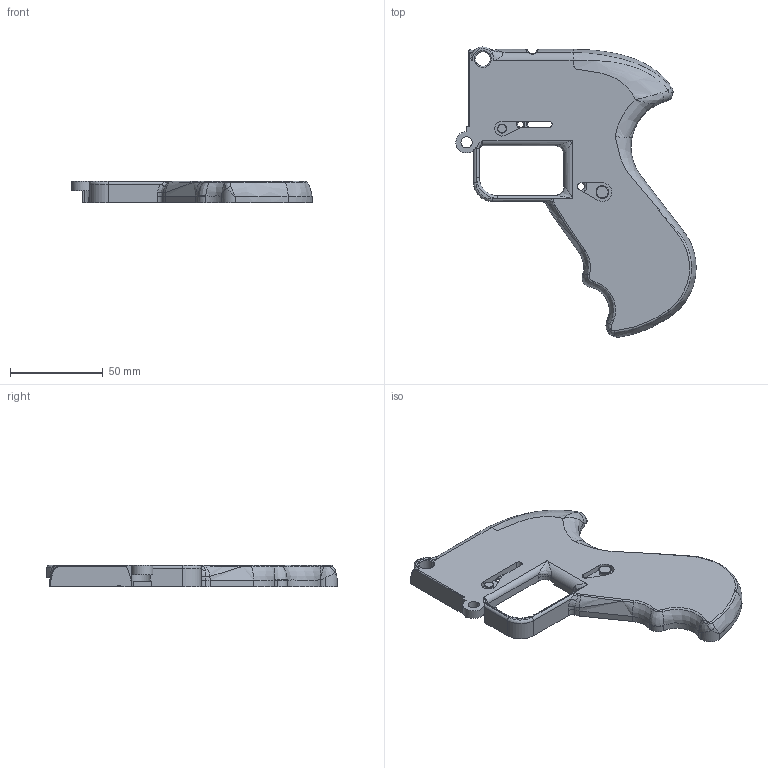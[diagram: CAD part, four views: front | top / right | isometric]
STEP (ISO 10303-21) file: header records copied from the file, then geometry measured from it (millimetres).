
FILE_DESCRIPTION (( 'STEP AP214' ), '1' );
FILE_NAME ('Imura_V3_Frame_Left.step', '2015-04-30T21:15:02', ( 'WarFairy' ), ( '' ), 'SwSTEP 2.0', 'SolidWorks 2013', '' );
FILE_SCHEMA (( 'AUTOMOTIVE_DESIGN' ));
Length unit declared in the file: millimetre
Products named in the file (1): Imura_V3_Frame_Left
Bounding box: 129.32 x 156.13 x 11.5 mm (x, y, z)
Volume: 71791.6 mm3; surface area: 30660.6 mm2
Topology: 1 solids, 1 shells, 246 faces, 686 edges, 444 vertices
Faces by surface type: cylinder 91, bspline 70, plane 64, torus 17, cone 4
Entity records: 14830 total; most frequent: CARTESIAN_POINT 8970, ORIENTED_EDGE 1370, DIRECTION 1064, EDGE_CURVE 685, VERTEX_POINT 444, AXIS2_PLACEMENT_3D 404, EDGE_LOOP 261, LINE 256
